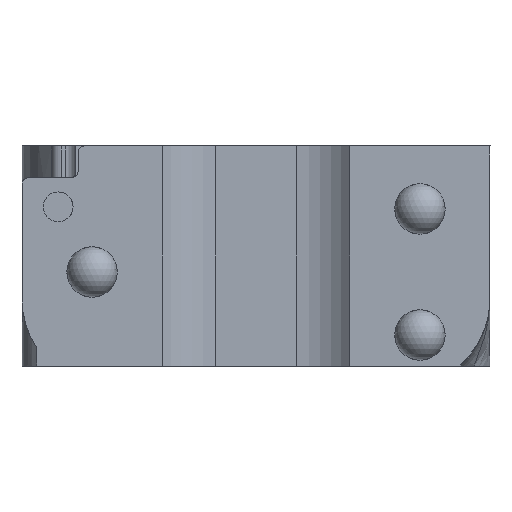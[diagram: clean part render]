
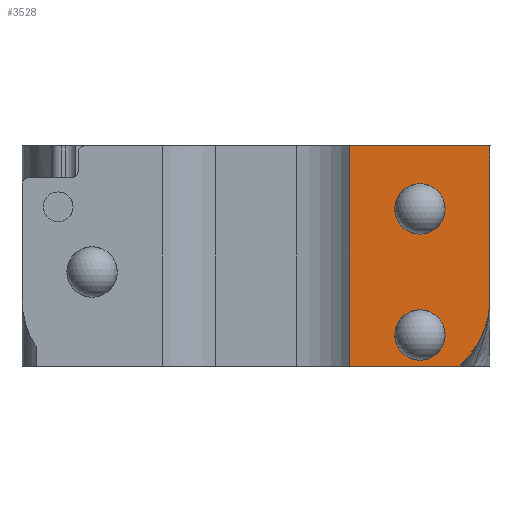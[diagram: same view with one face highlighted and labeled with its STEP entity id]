
A CAD part, left-side view. The second image highlights one B-rep face of the part: STEP entity #3528.
In plain terms, the highlighted planar face has unit normal (-1, 0, 0).
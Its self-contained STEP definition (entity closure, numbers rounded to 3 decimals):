
#40 = EDGE_CURVE ( 'NONE', #1464, #2296, #1264, .T. ) ;
#107 = EDGE_CURVE ( 'NONE', #2567, #1217, #1830, .T. ) ;
#146 = EDGE_CURVE ( 'NONE', #1217, #3351, #2721, .T. ) ;
#254 = EDGE_CURVE ( 'NONE', #3351, #3176, #3692, .T. ) ;
#404 = CARTESIAN_POINT ( 'NONE',  ( 82.199, -27.344, 8.815 ) ) ;
#409 = EDGE_CURVE ( 'NONE', #2105, #3176, #4941, .T. ) ;
#450 = EDGE_CURVE ( 'NONE', #2105, #2567, #1044, .T. ) ;
#639 = EDGE_CURVE ( 'NONE', #2503, #2976, #703, .T. ) ;
#670 = EDGE_CURVE ( 'NONE', #2976, #2503, #1528, .T. ) ;
#703 = CIRCLE ( 'NONE', #3514, 2. ) ;
#1044 = LINE ( 'NONE', #4149, #3055 ) ;
#1098 = CARTESIAN_POINT ( 'NONE',  ( 82.199, -30.901, 1.695 ) ) ;
#1217 = VERTEX_POINT ( 'NONE', #1098 ) ;
#1264 = CIRCLE ( 'NONE', #2759, 2. ) ;
#1380 = DIRECTION ( 'NONE',  ( 0., 1., 0. ) ) ;
#1382 = FACE_BOUND ( 'NONE', #3769, .T. ) ;
#1416 = DIRECTION ( 'NONE',  ( -1., 0., 0. ) ) ;
#1431 = CARTESIAN_POINT ( 'NONE',  ( 82.199, -25.344, 8.815 ) ) ;
#1464 = VERTEX_POINT ( 'NONE', #404 ) ;
#1528 = CIRCLE ( 'NONE', #2898, 2. ) ;
#1588 = ORIENTED_EDGE ( 'NONE', *, *, #40, .F. ) ;
#1830 = CIRCLE ( 'NONE', #1870, 7.057 ) ;
#1870 = AXIS2_PLACEMENT_3D ( 'NONE', #4704, #4701, #3572 ) ;
#1876 = DIRECTION ( 'NONE',  ( 0., 1., 0. ) ) ;
#1894 = CARTESIAN_POINT ( 'NONE',  ( 82.199, 69.175, 17.442 ) ) ;
#1897 = EDGE_LOOP ( 'NONE', ( #4625, #2208, #2192, #2226, #2237 ) ) ;
#1902 = PLANE ( 'NONE',  #5037 ) ;
#1912 = DIRECTION ( 'NONE',  ( 1., 0., 0. ) ) ;
#2105 = VERTEX_POINT ( 'NONE', #4924 ) ;
#2192 = ORIENTED_EDGE ( 'NONE', *, *, #254, .T. ) ;
#2208 = ORIENTED_EDGE ( 'NONE', *, *, #146, .T. ) ;
#2226 = ORIENTED_EDGE ( 'NONE', *, *, #409, .F. ) ;
#2237 = ORIENTED_EDGE ( 'NONE', *, *, #450, .T. ) ;
#2262 = ORIENTED_EDGE ( 'NONE', *, *, #639, .F. ) ;
#2272 = CARTESIAN_POINT ( 'NONE',  ( 82.199, -30.901, 13.815 ) ) ;
#2286 = ORIENTED_EDGE ( 'NONE', *, *, #670, .F. ) ;
#2296 = VERTEX_POINT ( 'NONE', #4392 ) ;
#2456 = CARTESIAN_POINT ( 'NONE',  ( 82.199, 1.953, 13.815 ) ) ;
#2503 = VERTEX_POINT ( 'NONE', #3820 ) ;
#2506 = DIRECTION ( 'NONE',  ( 0., 1., 0. ) ) ;
#2560 = CARTESIAN_POINT ( 'NONE',  ( 82.199, -19.787, 13.815 ) ) ;
#2567 = VERTEX_POINT ( 'NONE', #3758 ) ;
#2661 = VECTOR ( 'NONE', #4710, 1000. ) ;
#2668 = EDGE_LOOP ( 'NONE', ( #4574, #1588 ) ) ;
#2721 = LINE ( 'NONE', #3629, #2661 ) ;
#2759 = AXIS2_PLACEMENT_3D ( 'NONE', #4643, #4644, #4619 ) ;
#2857 = DIRECTION ( 'NONE',  ( 0., 1., 0. ) ) ;
#2867 = DIRECTION ( 'NONE',  ( -1., 0., 0. ) ) ;
#2870 = CARTESIAN_POINT ( 'NONE',  ( 82.199, -25.344, -1.185 ) ) ;
#2898 = AXIS2_PLACEMENT_3D ( 'NONE', #2870, #2867, #2857 ) ;
#2976 = VERTEX_POINT ( 'NONE', #3035 ) ;
#3035 = CARTESIAN_POINT ( 'NONE',  ( 82.199, -27.344, -1.185 ) ) ;
#3055 = VECTOR ( 'NONE', #4188, 1000. ) ;
#3129 = CIRCLE ( 'NONE', #3370, 2. ) ;
#3143 = DIRECTION ( 'NONE',  ( 0., 1., 0. ) ) ;
#3149 = DIRECTION ( 'NONE',  ( -1., 0., 0. ) ) ;
#3155 = CARTESIAN_POINT ( 'NONE',  ( 82.199, -25.344, -1.185 ) ) ;
#3176 = VERTEX_POINT ( 'NONE', #2560 ) ;
#3202 = VECTOR ( 'NONE', #2506, 1000. ) ;
#3351 = VERTEX_POINT ( 'NONE', #2272 ) ;
#3370 = AXIS2_PLACEMENT_3D ( 'NONE', #1431, #1416, #1380 ) ;
#3513 = FACE_OUTER_BOUND ( 'NONE', #1897, .T. ) ;
#3514 = AXIS2_PLACEMENT_3D ( 'NONE', #3155, #3149, #3143 ) ;
#3528 = ADVANCED_FACE ( 'NONE', ( #4519, #3513, #1382 ), #1902, .F. ) ;
#3572 = DIRECTION ( 'NONE',  ( 0., 1., 0. ) ) ;
#3629 = CARTESIAN_POINT ( 'NONE',  ( 82.199, -30.901, 1.695 ) ) ;
#3692 = LINE ( 'NONE', #2456, #3202 ) ;
#3758 = CARTESIAN_POINT ( 'NONE',  ( 82.199, -28.455, -3.647 ) ) ;
#3769 = EDGE_LOOP ( 'NONE', ( #2262, #2286 ) ) ;
#3820 = CARTESIAN_POINT ( 'NONE',  ( 82.199, -23.344, -1.185 ) ) ;
#4149 = CARTESIAN_POINT ( 'NONE',  ( 82.199, 69.175, -3.647 ) ) ;
#4188 = DIRECTION ( 'NONE',  ( 0., -1., 0. ) ) ;
#4207 = VECTOR ( 'NONE', #4380, 1000. ) ;
#4380 = DIRECTION ( 'NONE',  ( 0., 0., 1. ) ) ;
#4385 = CARTESIAN_POINT ( 'NONE',  ( 82.199, -19.787, -17.935 ) ) ;
#4392 = CARTESIAN_POINT ( 'NONE',  ( 82.199, -23.344, 8.815 ) ) ;
#4519 = FACE_BOUND ( 'NONE', #2668, .T. ) ;
#4574 = ORIENTED_EDGE ( 'NONE', *, *, #5100, .F. ) ;
#4619 = DIRECTION ( 'NONE',  ( 0., 1., 0. ) ) ;
#4625 = ORIENTED_EDGE ( 'NONE', *, *, #107, .T. ) ;
#4643 = CARTESIAN_POINT ( 'NONE',  ( 82.199, -25.344, 8.815 ) ) ;
#4644 = DIRECTION ( 'NONE',  ( -1., 0., 0. ) ) ;
#4701 = DIRECTION ( 'NONE',  ( -1., 0., 0. ) ) ;
#4704 = CARTESIAN_POINT ( 'NONE',  ( 82.199, -23.844, 1.695 ) ) ;
#4710 = DIRECTION ( 'NONE',  ( 0., 0., 1. ) ) ;
#4924 = CARTESIAN_POINT ( 'NONE',  ( 82.199, -19.787, -3.647 ) ) ;
#4941 = LINE ( 'NONE', #4385, #4207 ) ;
#5037 = AXIS2_PLACEMENT_3D ( 'NONE', #1894, #1912, #1876 ) ;
#5100 = EDGE_CURVE ( 'NONE', #2296, #1464, #3129, .T. ) ;
